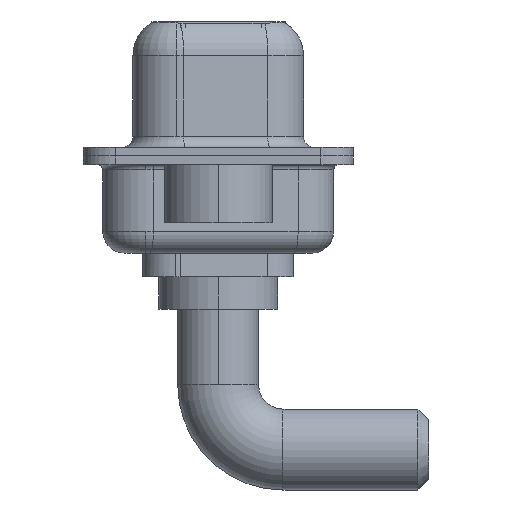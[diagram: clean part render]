
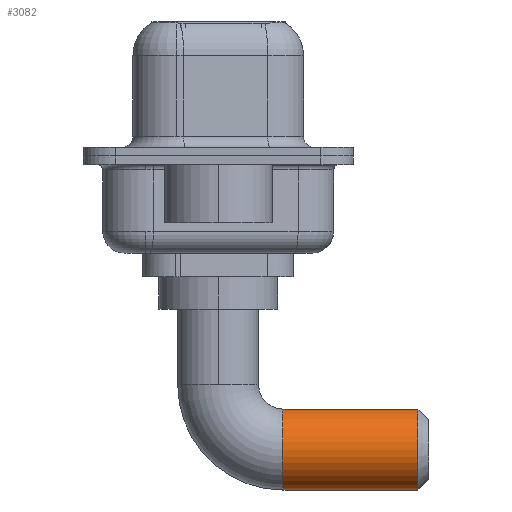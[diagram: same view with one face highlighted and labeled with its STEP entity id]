
A CAD part, left-side view. The second image highlights one B-rep face of the part: STEP entity #3082.
In plain terms, the highlighted cylindrical face has radius 1.875 mm (diameter 3.75 mm), a partial arc.
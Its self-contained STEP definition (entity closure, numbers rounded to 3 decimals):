
#78 = VERTEX_POINT ( 'NONE', #6090 ) ;
#341 = AXIS2_PLACEMENT_3D ( 'NONE', #2130, #11307, #4461 ) ;
#390 = LINE ( 'NONE', #8641, #4928 ) ;
#728 = ORIENTED_EDGE ( 'NONE', *, *, #878, .T. ) ;
#878 = EDGE_CURVE ( 'NONE', #3325, #78, #11545, .T. ) ;
#1045 = CARTESIAN_POINT ( 'NONE',  ( 0., -3., -8.375 ) ) ;
#1879 = DIRECTION ( 'NONE',  ( 0., 0., -1. ) ) ;
#1918 = CARTESIAN_POINT ( 'NONE',  ( 0., -9.25, -6.5 ) ) ;
#1942 = CYLINDRICAL_SURFACE ( 'NONE', #13022, 1.875 ) ;
#2130 = CARTESIAN_POINT ( 'NONE',  ( 0., -3., -6.5 ) ) ;
#2534 = DIRECTION ( 'NONE',  ( 0., -1., 0. ) ) ;
#3082 = ADVANCED_FACE ( 'NONE', ( #6846 ), #1942, .T. ) ;
#3325 = VERTEX_POINT ( 'NONE', #12734 ) ;
#3385 = EDGE_CURVE ( 'NONE', #3642, #78, #390, .T. ) ;
#3642 = VERTEX_POINT ( 'NONE', #5069 ) ;
#4461 = DIRECTION ( 'NONE',  ( -1., 0., 0. ) ) ;
#4677 = AXIS2_PLACEMENT_3D ( 'NONE', #1918, #11298, #6075 ) ;
#4928 = VECTOR ( 'NONE', #2534, 1000. ) ;
#5069 = CARTESIAN_POINT ( 'NONE',  ( 0., -3., -4.625 ) ) ;
#5274 = EDGE_CURVE ( 'NONE', #5570, #3325, #12820, .T. ) ;
#5570 = VERTEX_POINT ( 'NONE', #1045 ) ;
#6075 = DIRECTION ( 'NONE',  ( 0., 0., -1. ) ) ;
#6090 = CARTESIAN_POINT ( 'NONE',  ( 0., -9.25, -4.625 ) ) ;
#6724 = CARTESIAN_POINT ( 'NONE',  ( 0., -3., -8.375 ) ) ;
#6846 = FACE_OUTER_BOUND ( 'NONE', #8734, .T. ) ;
#7982 = VECTOR ( 'NONE', #8727, 1000. ) ;
#8641 = CARTESIAN_POINT ( 'NONE',  ( 0., -3., -4.625 ) ) ;
#8727 = DIRECTION ( 'NONE',  ( 0., -1., 0. ) ) ;
#8734 = EDGE_LOOP ( 'NONE', ( #8895, #9545, #8973, #728 ) ) ;
#8855 = DIRECTION ( 'NONE',  ( 0., -1., 0. ) ) ;
#8895 = ORIENTED_EDGE ( 'NONE', *, *, #3385, .F. ) ;
#8973 = ORIENTED_EDGE ( 'NONE', *, *, #5274, .T. ) ;
#9545 = ORIENTED_EDGE ( 'NONE', *, *, #10226, .T. ) ;
#9935 = CARTESIAN_POINT ( 'NONE',  ( 0., -3., -6.5 ) ) ;
#10226 = EDGE_CURVE ( 'NONE', #3642, #5570, #12552, .T. ) ;
#11298 = DIRECTION ( 'NONE',  ( 0., 1., 0. ) ) ;
#11307 = DIRECTION ( 'NONE',  ( 0., -1., 0. ) ) ;
#11545 = CIRCLE ( 'NONE', #4677, 1.875 ) ;
#12552 = CIRCLE ( 'NONE', #341, 1.875 ) ;
#12734 = CARTESIAN_POINT ( 'NONE',  ( 0., -9.25, -8.375 ) ) ;
#12820 = LINE ( 'NONE', #6724, #7982 ) ;
#13022 = AXIS2_PLACEMENT_3D ( 'NONE', #9935, #8855, #1879 ) ;
